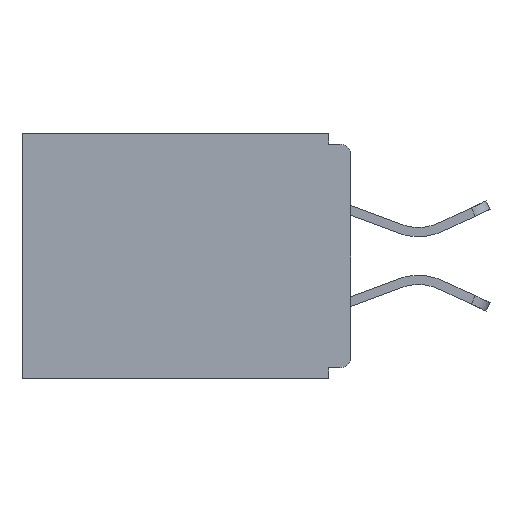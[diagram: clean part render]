
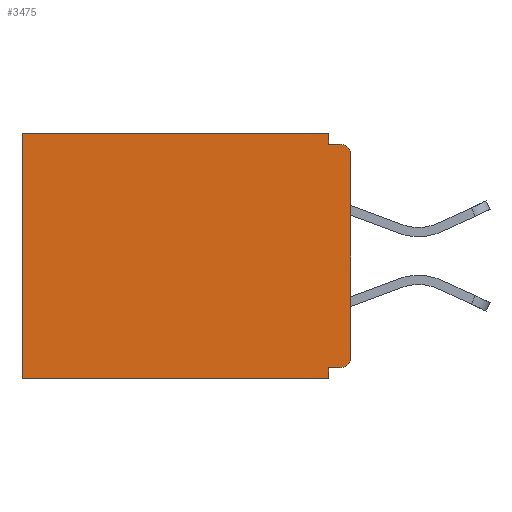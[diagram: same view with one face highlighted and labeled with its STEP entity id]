
A CAD part, left-side view. The second image highlights one B-rep face of the part: STEP entity #3475.
In plain terms, the highlighted planar face has unit normal (-1, 0, 0).
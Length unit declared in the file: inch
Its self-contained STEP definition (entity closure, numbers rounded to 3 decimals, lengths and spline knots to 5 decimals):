
#353 = VERTEX_POINT ( 'NONE', #20433 ) ;
#414 = CARTESIAN_POINT ( 'NONE',  ( 0.298, 0.031, -0.015 ) ) ;
#749 = CARTESIAN_POINT ( 'NONE',  ( 0.298, 0., -0.015 ) ) ;
#1383 = ORIENTED_EDGE ( 'NONE', *, *, #9369, .T. ) ;
#1461 = VECTOR ( 'NONE', #12728, 39.37008 ) ;
#1727 = CARTESIAN_POINT ( 'NONE',  ( 0.298, 0.015, -0.313 ) ) ;
#1932 = VECTOR ( 'NONE', #12062, 39.37008 ) ;
#1935 = VECTOR ( 'NONE', #15301, 39.37008 ) ;
#1946 = ORIENTED_EDGE ( 'NONE', *, *, #20406, .F. ) ;
#2227 = VECTOR ( 'NONE', #6606, 39.37008 ) ;
#2250 = CARTESIAN_POINT ( 'NONE',  ( 0.298, 0., -0.03 ) ) ;
#2640 = CARTESIAN_POINT ( 'NONE',  ( 0.298, 0., 0. ) ) ;
#2788 = CARTESIAN_POINT ( 'NONE',  ( 0.298, 0.031, 0. ) ) ;
#3475 = ADVANCED_FACE ( 'NONE', ( #5649 ), #5075, .F. ) ;
#3478 = CARTESIAN_POINT ( 'NONE',  ( 0.298, 0.031, -0.328 ) ) ;
#5039 = CARTESIAN_POINT ( 'NONE',  ( 0.298, 0., -0.328 ) ) ;
#5075 = PLANE ( 'NONE',  #6792 ) ;
#5115 = LINE ( 'NONE', #2640, #1935 ) ;
#5181 = EDGE_CURVE ( 'NONE', #14012, #12519, #7064, .T. ) ;
#5528 = VERTEX_POINT ( 'NONE', #20361 ) ;
#5649 = FACE_OUTER_BOUND ( 'NONE', #16435, .T. ) ;
#5838 = EDGE_CURVE ( 'NONE', #12986, #20363, #13033, .T. ) ;
#6097 = LINE ( 'NONE', #10799, #11550 ) ;
#6606 = DIRECTION ( 'NONE',  ( 0., 1., 0. ) ) ;
#6792 = AXIS2_PLACEMENT_3D ( 'NONE', #8468, #19548, #11469 ) ;
#6918 = ORIENTED_EDGE ( 'NONE', *, *, #16312, .F. ) ;
#7064 = LINE ( 'NONE', #18503, #1932 ) ;
#7968 = CARTESIAN_POINT ( 'NONE',  ( 0.298, 0., -0.313 ) ) ;
#8108 = VERTEX_POINT ( 'NONE', #2250 ) ;
#8279 = VERTEX_POINT ( 'NONE', #7968 ) ;
#8468 = CARTESIAN_POINT ( 'NONE',  ( 0.298, 0., 0. ) ) ;
#8608 = LINE ( 'NONE', #749, #17023 ) ;
#8785 = DIRECTION ( 'NONE',  ( 0., 0., -1. ) ) ;
#9369 = EDGE_CURVE ( 'NONE', #353, #8279, #11383, .T. ) ;
#10799 = CARTESIAN_POINT ( 'NONE',  ( 0.298, 0., -0.343 ) ) ;
#10835 = ORIENTED_EDGE ( 'NONE', *, *, #5838, .F. ) ;
#10921 = EDGE_CURVE ( 'NONE', #8108, #8279, #5115, .T. ) ;
#11136 = CARTESIAN_POINT ( 'NONE',  ( 0.298, 0.031, -0.343 ) ) ;
#11383 = CIRCLE ( 'NONE', #16507, 0.015 ) ;
#11418 = VECTOR ( 'NONE', #16821, 39.37008 ) ;
#11469 = DIRECTION ( 'NONE',  ( 0., 0., -1. ) ) ;
#11550 = VECTOR ( 'NONE', #12176, 39.37008 ) ;
#11880 = CARTESIAN_POINT ( 'NONE',  ( 0.298, 0.015, -0.03 ) ) ;
#12062 = DIRECTION ( 'NONE',  ( 0., 0., -1. ) ) ;
#12176 = DIRECTION ( 'NONE',  ( 0., 1., 0. ) ) ;
#12519 = VERTEX_POINT ( 'NONE', #414 ) ;
#12728 = DIRECTION ( 'NONE',  ( 0., 0., -1. ) ) ;
#12826 = DIRECTION ( 'NONE',  ( 0., 0., -1. ) ) ;
#12986 = VERTEX_POINT ( 'NONE', #3478 ) ;
#13033 = LINE ( 'NONE', #11136, #1461 ) ;
#13087 = CARTESIAN_POINT ( 'NONE',  ( 0.298, 0.031, -0.343 ) ) ;
#13159 = ORIENTED_EDGE ( 'NONE', *, *, #10921, .F. ) ;
#13340 = AXIS2_PLACEMENT_3D ( 'NONE', #11880, #18258, #8785 ) ;
#13598 = ORIENTED_EDGE ( 'NONE', *, *, #18340, .T. ) ;
#13792 = EDGE_CURVE ( 'NONE', #5528, #15601, #18845, .T. ) ;
#14012 = VERTEX_POINT ( 'NONE', #2788 ) ;
#14639 = ORIENTED_EDGE ( 'NONE', *, *, #19256, .T. ) ;
#14797 = LINE ( 'NONE', #5039, #2227 ) ;
#15090 = VECTOR ( 'NONE', #15787, 39.37008 ) ;
#15097 = EDGE_CURVE ( 'NONE', #353, #12986, #14797, .T. ) ;
#15301 = DIRECTION ( 'NONE',  ( 0., 0., -1. ) ) ;
#15431 = ORIENTED_EDGE ( 'NONE', *, *, #15097, .F. ) ;
#15601 = VERTEX_POINT ( 'NONE', #15607 ) ;
#15607 = CARTESIAN_POINT ( 'NONE',  ( 0.298, 0.46, -0.343 ) ) ;
#15787 = DIRECTION ( 'NONE',  ( 0., 1., 0. ) ) ;
#15833 = DIRECTION ( 'NONE',  ( -1., 0., 0. ) ) ;
#15925 = ORIENTED_EDGE ( 'NONE', *, *, #5181, .F. ) ;
#16312 = EDGE_CURVE ( 'NONE', #20363, #15601, #6097, .T. ) ;
#16326 = VERTEX_POINT ( 'NONE', #17297 ) ;
#16435 = EDGE_LOOP ( 'NONE', ( #14639, #1946, #15925, #13598, #17245, #6918, #10835, #15431, #1383, #13159 ) ) ;
#16507 = AXIS2_PLACEMENT_3D ( 'NONE', #1727, #15833, #12826 ) ;
#16524 = CIRCLE ( 'NONE', #13340, 0.015 ) ;
#16821 = DIRECTION ( 'NONE',  ( 0., 0., -1. ) ) ;
#17023 = VECTOR ( 'NONE', #18118, 39.37008 ) ;
#17245 = ORIENTED_EDGE ( 'NONE', *, *, #13792, .T. ) ;
#17297 = CARTESIAN_POINT ( 'NONE',  ( 0.298, 0.015, -0.015 ) ) ;
#17323 = CARTESIAN_POINT ( 'NONE',  ( 0.298, 0., 0. ) ) ;
#18118 = DIRECTION ( 'NONE',  ( 0., -1., 0. ) ) ;
#18258 = DIRECTION ( 'NONE',  ( -1., 0., 0. ) ) ;
#18340 = EDGE_CURVE ( 'NONE', #14012, #5528, #19343, .T. ) ;
#18455 = CARTESIAN_POINT ( 'NONE',  ( 0.298, 0.46, 0. ) ) ;
#18503 = CARTESIAN_POINT ( 'NONE',  ( 0.298, 0.031, -0.343 ) ) ;
#18845 = LINE ( 'NONE', #18455, #11418 ) ;
#19256 = EDGE_CURVE ( 'NONE', #8108, #16326, #16524, .T. ) ;
#19343 = LINE ( 'NONE', #17323, #15090 ) ;
#19548 = DIRECTION ( 'NONE',  ( 1., 0., 0. ) ) ;
#20361 = CARTESIAN_POINT ( 'NONE',  ( 0.298, 0.46, 0. ) ) ;
#20363 = VERTEX_POINT ( 'NONE', #13087 ) ;
#20406 = EDGE_CURVE ( 'NONE', #12519, #16326, #8608, .T. ) ;
#20433 = CARTESIAN_POINT ( 'NONE',  ( 0.298, 0.015, -0.328 ) ) ;
